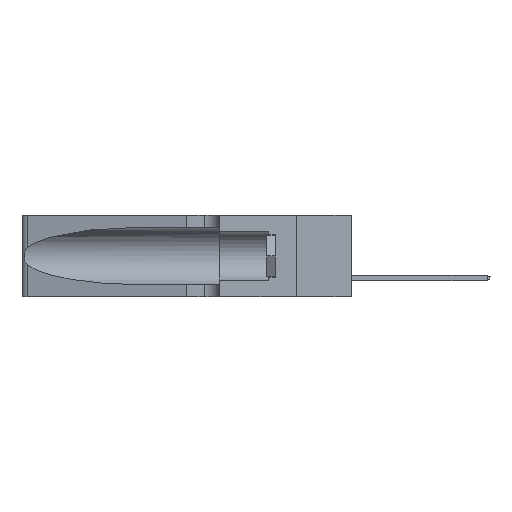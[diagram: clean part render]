
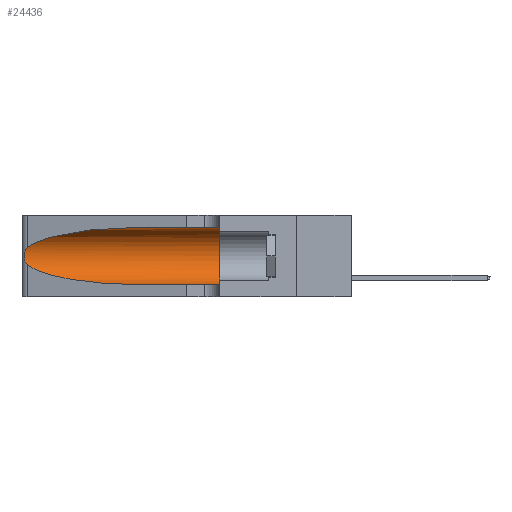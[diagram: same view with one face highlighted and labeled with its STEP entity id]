
A CAD part, left-side view. The second image highlights one B-rep face of the part: STEP entity #24436.
In plain terms, the highlighted cylindrical face has radius 3.308 mm (diameter 6.617 mm), a partial arc.
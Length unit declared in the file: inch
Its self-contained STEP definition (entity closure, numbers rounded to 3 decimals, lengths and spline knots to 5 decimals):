
#51 = ORIENTED_EDGE ( 'NONE', *, *, #14024, .F. ) ;
#334 = EDGE_CURVE ( 'NONE', #39384, #25054, #46281, .T. ) ;
#1169 = DIRECTION ( 'NONE',  ( 0., 1., 0. ) ) ;
#1343 = CARTESIAN_POINT ( 'NONE',  ( 0.25487, 1.22718, 0.14631 ) ) ;
#1552 = CARTESIAN_POINT ( 'NONE',  ( 0.26075, 1.23896, 0.178 ) ) ;
#1725 = CARTESIAN_POINT ( 'NONE',  ( 0.25789, 1.23486, 0.15765 ) ) ;
#2256 = CARTESIAN_POINT ( 'NONE',  ( 0.25487, 1.22718, 0.22369 ) ) ;
#3317 = CARTESIAN_POINT ( 'NONE',  ( 0.25487, 1.22718, 0.14631 ) ) ;
#3843 = EDGE_CURVE ( 'NONE', #7160, #39384, #19658, .T. ) ;
#4741 = CARTESIAN_POINT ( 'NONE',  ( 0.1305, 0.72297, 0.05475 ) ) ;
#5086 = CARTESIAN_POINT ( 'NONE',  ( 0.25555, 1.22994, 0.2215 ) ) ;
#5278 = VERTEX_POINT ( 'NONE', #27842 ) ;
#5751 = CARTESIAN_POINT ( 'NONE',  ( 0.18966, 0.96281, 0.31525 ) ) ;
#5948 = EDGE_LOOP ( 'NONE', ( #32901, #31265, #10110, #27755, #51, #40423 ) ) ;
#7160 = VERTEX_POINT ( 'NONE', #3317 ) ;
#8242 = CARTESIAN_POINT ( 'NONE',  ( 0.25487, 1.22718, 0.22369 ) ) ;
#9118 = CARTESIAN_POINT ( 'NONE',  ( 0.1305, 0.72297, 0.05475 ) ) ;
#9234 = CARTESIAN_POINT ( 'NONE',  ( 0.25487, 1.22718, 0.14631 ) ) ;
#9553 = VECTOR ( 'NONE', #32522, 39.37008 ) ;
#10110 = ORIENTED_EDGE ( 'NONE', *, *, #3843, .T. ) ;
#10251 = CARTESIAN_POINT ( 'NONE',  ( 0.1305, 1.61858, 0.185 ) ) ;
#13556 = B_SPLINE_CURVE_WITH_KNOTS ( 'NONE', 3,
 ( #33849, #5086, #37653, #19187, #16053, #41275, #33517, #1552, #44867, #38305, #1725, #23621, #34686, #9234 ),
 .UNSPECIFIED., .F., .F.,
 ( 4, 2, 2, 2, 2, 2, 4 ),
 ( 0., 0.00027, 0.00053, 0.00107, 0.0016, 0.00187, 0.00214 ),
 .UNSPECIFIED. ) ;
#13912 = DIRECTION ( 'NONE',  ( 0., 0., -1. ) ) ;
#14024 = EDGE_CURVE ( 'NONE', #5278, #25054, #38330, .T. ) ;
#14043 = CARTESIAN_POINT ( 'NONE',  ( 0.1305, 0.72297, 0.31525 ) ) ;
#15246 = FACE_OUTER_BOUND ( 'NONE', #5948, .T. ) ;
#16053 = CARTESIAN_POINT ( 'NONE',  ( 0.25854, 1.2359, 0.20912 ) ) ;
#16092 = EDGE_CURVE ( 'NONE', #16940, #5278, #31919, .T. ) ;
#16940 = VERTEX_POINT ( 'NONE', #14043 ) ;
#18321 = CARTESIAN_POINT ( 'NONE',  ( 0.1305, 1.61858, 0.05475 ) ) ;
#19187 = CARTESIAN_POINT ( 'NONE',  ( 0.25787, 1.23484, 0.2124 ) ) ;
#19300 = CARTESIAN_POINT ( 'NONE',  ( 0.1305, 0.35, 0.185 ) ) ;
#19658 =( BOUNDED_CURVE ( )  B_SPLINE_CURVE ( 3, ( #1343, #29861, #26543, #4741 ),
 .UNSPECIFIED., .F., .T. ) 
 B_SPLINE_CURVE_WITH_KNOTS ( ( 4, 4 ),
 ( 3.44316, 4.71239 ),
 .UNSPECIFIED. ) 
 CURVE ( )  GEOMETRIC_REPRESENTATION_ITEM ( )  RATIONAL_B_SPLINE_CURVE ( ( 1., 0.87, 0.87, 1. ) ) 
 REPRESENTATION_ITEM ( '' )  );
#19908 = CARTESIAN_POINT ( 'NONE',  ( 0.1305, 0.35, 0.05475 ) ) ;
#20543 = AXIS2_PLACEMENT_3D ( 'NONE', #19300, #1169, #23409 ) ;
#23409 = DIRECTION ( 'NONE',  ( 0., 0., 1. ) ) ;
#23474 = CARTESIAN_POINT ( 'NONE',  ( 0.1305, 0.72297, 0.31525 ) ) ;
#23621 = CARTESIAN_POINT ( 'NONE',  ( 0.25639, 1.23186, 0.15144 ) ) ;
#24150 = DIRECTION ( 'NONE',  ( 0., -1., 0. ) ) ;
#24436 = ADVANCED_FACE ( 'NONE', ( #15246 ), #41226, .F. ) ;
#25054 = VERTEX_POINT ( 'NONE', #19908 ) ;
#26543 = CARTESIAN_POINT ( 'NONE',  ( 0.18966, 0.96281, 0.05475 ) ) ;
#27755 = ORIENTED_EDGE ( 'NONE', *, *, #334, .T. ) ;
#27842 = CARTESIAN_POINT ( 'NONE',  ( 0.1305, 0.35, 0.31525 ) ) ;
#29473 =( BOUNDED_CURVE ( )  B_SPLINE_CURVE ( 3, ( #23474, #5751, #38335, #2256 ),
 .UNSPECIFIED., .F., .F. ) 
 B_SPLINE_CURVE_WITH_KNOTS ( ( 4, 4 ),
 ( 1.5708, 2.84003 ),
 .UNSPECIFIED. ) 
 CURVE ( )  GEOMETRIC_REPRESENTATION_ITEM ( )  RATIONAL_B_SPLINE_CURVE ( ( 1., 0.87, 0.87, 1. ) ) 
 REPRESENTATION_ITEM ( '' )  );
#29861 = CARTESIAN_POINT ( 'NONE',  ( 0.2373, 1.15595, 0.08982 ) ) ;
#31265 = ORIENTED_EDGE ( 'NONE', *, *, #46445, .T. ) ;
#31919 = LINE ( 'NONE', #45053, #39779 ) ;
#32522 = DIRECTION ( 'NONE',  ( 0., -1., 0. ) ) ;
#32901 = ORIENTED_EDGE ( 'NONE', *, *, #34220, .T. ) ;
#33517 = CARTESIAN_POINT ( 'NONE',  ( 0.26075, 1.23896, 0.19203 ) ) ;
#33815 = VERTEX_POINT ( 'NONE', #8242 ) ;
#33849 = CARTESIAN_POINT ( 'NONE',  ( 0.25487, 1.22718, 0.22369 ) ) ;
#34220 = EDGE_CURVE ( 'NONE', #16940, #33815, #29473, .T. ) ;
#34267 = AXIS2_PLACEMENT_3D ( 'NONE', #10251, #24150, #13912 ) ;
#34686 = CARTESIAN_POINT ( 'NONE',  ( 0.25555, 1.22993, 0.14849 ) ) ;
#37653 = CARTESIAN_POINT ( 'NONE',  ( 0.25639, 1.23184, 0.21858 ) ) ;
#38305 = CARTESIAN_POINT ( 'NONE',  ( 0.25856, 1.23593, 0.16098 ) ) ;
#38330 = CIRCLE ( 'NONE', #20543, 0.13025 ) ;
#38335 = CARTESIAN_POINT ( 'NONE',  ( 0.2373, 1.15595, 0.28018 ) ) ;
#39384 = VERTEX_POINT ( 'NONE', #9118 ) ;
#39779 = VECTOR ( 'NONE', #41940, 39.37008 ) ;
#40423 = ORIENTED_EDGE ( 'NONE', *, *, #16092, .F. ) ;
#41226 = CYLINDRICAL_SURFACE ( 'NONE', #34267, 0.13025 ) ;
#41275 = CARTESIAN_POINT ( 'NONE',  ( 0.26018, 1.23835, 0.19895 ) ) ;
#41940 = DIRECTION ( 'NONE',  ( 0., -1., 0. ) ) ;
#44867 = CARTESIAN_POINT ( 'NONE',  ( 0.26017, 1.23833, 0.17102 ) ) ;
#45053 = CARTESIAN_POINT ( 'NONE',  ( 0.1305, 1.61858, 0.31525 ) ) ;
#46281 = LINE ( 'NONE', #18321, #9553 ) ;
#46445 = EDGE_CURVE ( 'NONE', #33815, #7160, #13556, .T. ) ;
